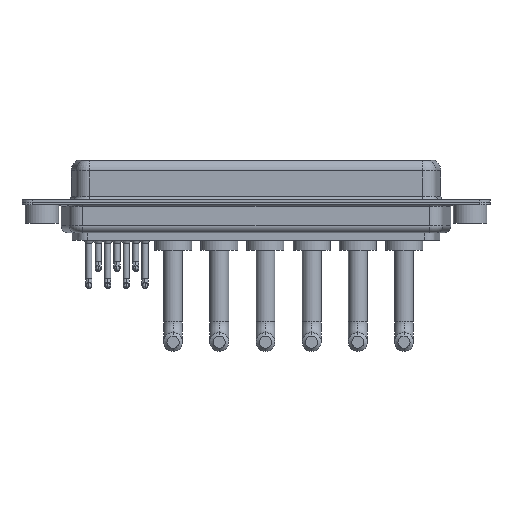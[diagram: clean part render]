
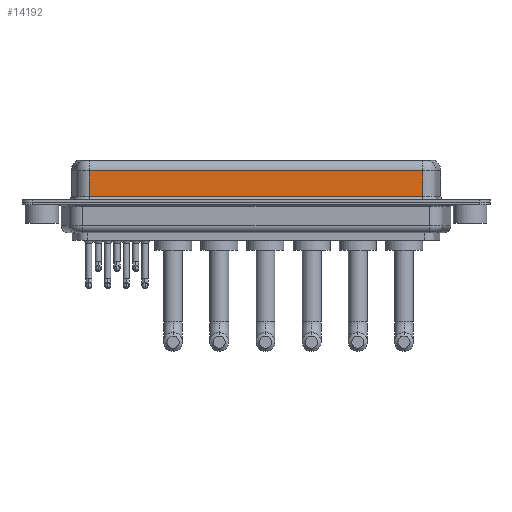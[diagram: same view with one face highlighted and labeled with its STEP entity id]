
A CAD part, front view. The second image highlights one B-rep face of the part: STEP entity #14192.
In plain terms, the highlighted planar face has unit normal (0, -1, 0).
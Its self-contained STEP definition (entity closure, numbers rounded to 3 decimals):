
#4 = DIRECTION ( 'NONE',  ( 0., 0., 1. ) ) ;
#1034 = VERTEX_POINT ( 'NONE', #6638 ) ;
#2145 = VECTOR ( 'NONE', #9238, 1000. ) ;
#2253 = DIRECTION ( 'NONE',  ( 1., 0., 0. ) ) ;
#2662 = EDGE_CURVE ( 'NONE', #11791, #7089, #13524, .T. ) ;
#2802 = ORIENTED_EDGE ( 'NONE', *, *, #12829, .T. ) ;
#4420 = VERTEX_POINT ( 'NONE', #7013 ) ;
#5134 = LINE ( 'NONE', #7828, #9626 ) ;
#5415 = CARTESIAN_POINT ( 'NONE',  ( 7.038, -3.95, 6.4 ) ) ;
#5817 = CARTESIAN_POINT ( 'NONE',  ( 56.462, -3.95, 4.65 ) ) ;
#6638 = CARTESIAN_POINT ( 'NONE',  ( 7.038, -3.95, 0.9 ) ) ;
#7013 = CARTESIAN_POINT ( 'NONE',  ( 56.462, -3.95, 0.9 ) ) ;
#7089 = VERTEX_POINT ( 'NONE', #10823 ) ;
#7388 = CARTESIAN_POINT ( 'NONE',  ( 56.462, -3.95, 6.4 ) ) ;
#7828 = CARTESIAN_POINT ( 'NONE',  ( 56.462, -3.95, 0.9 ) ) ;
#8298 = PLANE ( 'NONE',  #11701 ) ;
#9238 = DIRECTION ( 'NONE',  ( -1., 0., 0. ) ) ;
#9626 = VECTOR ( 'NONE', #2253, 1000. ) ;
#10823 = CARTESIAN_POINT ( 'NONE',  ( 7.038, -3.95, 4.65 ) ) ;
#11687 = DIRECTION ( 'NONE',  ( 0., 0., -1. ) ) ;
#11701 = AXIS2_PLACEMENT_3D ( 'NONE', #12771, #15458, #4 ) ;
#11791 = VERTEX_POINT ( 'NONE', #15248 ) ;
#12371 = ORIENTED_EDGE ( 'NONE', *, *, #2662, .T. ) ;
#12771 = CARTESIAN_POINT ( 'NONE',  ( 56.462, -3.95, 6.4 ) ) ;
#12829 = EDGE_CURVE ( 'NONE', #7089, #1034, #15370, .T. ) ;
#13524 = LINE ( 'NONE', #5817, #2145 ) ;
#13816 = VECTOR ( 'NONE', #11687, 1000. ) ;
#14071 = DIRECTION ( 'NONE',  ( 0., 0., -1. ) ) ;
#14103 = EDGE_CURVE ( 'NONE', #1034, #4420, #5134, .T. ) ;
#14192 = ADVANCED_FACE ( 'NONE', ( #18334 ), #8298, .F. ) ;
#15134 = EDGE_CURVE ( 'NONE', #11791, #4420, #16993, .T. ) ;
#15248 = CARTESIAN_POINT ( 'NONE',  ( 56.462, -3.95, 4.65 ) ) ;
#15370 = LINE ( 'NONE', #5415, #17299 ) ;
#15458 = DIRECTION ( 'NONE',  ( 0., 1., 0. ) ) ;
#16358 = ORIENTED_EDGE ( 'NONE', *, *, #15134, .F. ) ;
#16993 = LINE ( 'NONE', #7388, #13816 ) ;
#17299 = VECTOR ( 'NONE', #14071, 1000. ) ;
#17429 = EDGE_LOOP ( 'NONE', ( #16358, #12371, #2802, #17711 ) ) ;
#17711 = ORIENTED_EDGE ( 'NONE', *, *, #14103, .T. ) ;
#18334 = FACE_OUTER_BOUND ( 'NONE', #17429, .T. ) ;
